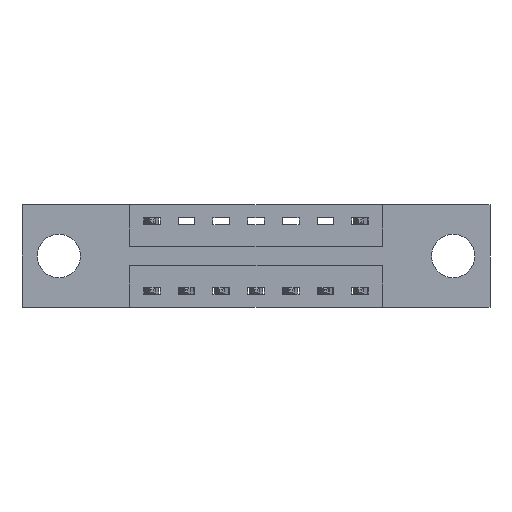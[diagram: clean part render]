
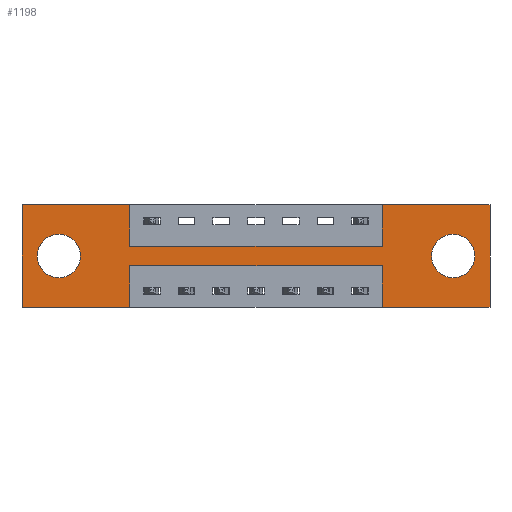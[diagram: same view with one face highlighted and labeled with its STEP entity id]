
A CAD part, front view. The second image highlights one B-rep face of the part: STEP entity #1198.
In plain terms, the highlighted planar face has unit normal (0, -1, 0).
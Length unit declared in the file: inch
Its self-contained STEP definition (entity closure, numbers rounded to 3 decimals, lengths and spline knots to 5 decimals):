
#20 = CARTESIAN_POINT ( 'NONE',  ( 1.5525, 0., -0.185 ) ) ;
#80 = CARTESIAN_POINT ( 'NONE',  ( 0.3875, 0., 0. ) ) ;
#141 = FACE_BOUND ( 'NONE', #5571, .T. ) ;
#266 = EDGE_LOOP ( 'NONE', ( #6934, #7665, #6947, #8512, #7149, #7156, #8659, #7692, #7305, #8444, #7357, #8409 ) ) ;
#296 = DIRECTION ( 'NONE',  ( 0., 1., 0. ) ) ;
#510 = LINE ( 'NONE', #8257, #4146 ) ;
#536 = DIRECTION ( 'NONE',  ( -1., 0., 0. ) ) ;
#577 = VERTEX_POINT ( 'NONE', #8820 ) ;
#596 = LINE ( 'NONE', #5218, #8193 ) ;
#825 = AXIS2_PLACEMENT_3D ( 'NONE', #4644, #296, #5384 ) ;
#826 = DIRECTION ( 'NONE',  ( 0., 0., -1. ) ) ;
#847 = EDGE_CURVE ( 'NONE', #7446, #1345, #1660, .T. ) ;
#893 = DIRECTION ( 'NONE',  ( 0., 0., -1. ) ) ;
#1031 = CARTESIAN_POINT ( 'NONE',  ( 1.2975, 0., -0.22 ) ) ;
#1149 = VERTEX_POINT ( 'NONE', #3296 ) ;
#1194 = EDGE_CURVE ( 'NONE', #7522, #4531, #8883, .T. ) ;
#1198 = ADVANCED_FACE ( 'NONE', ( #141, #7212, #3389 ), #7716, .T. ) ;
#1345 = VERTEX_POINT ( 'NONE', #2401 ) ;
#1363 = DIRECTION ( 'NONE',  ( 0., -1., 0. ) ) ;
#1406 = VECTOR ( 'NONE', #2763, 39.37008 ) ;
#1538 = EDGE_CURVE ( 'NONE', #577, #3326, #7720, .T. ) ;
#1622 = CARTESIAN_POINT ( 'NONE',  ( 0.3875, 0., -0.15 ) ) ;
#1660 = CIRCLE ( 'NONE', #1669, 0.078 ) ;
#1669 = AXIS2_PLACEMENT_3D ( 'NONE', #3978, #8791, #4691 ) ;
#1835 = DIRECTION ( 'NONE',  ( -1., 0., 0. ) ) ;
#2041 = AXIS2_PLACEMENT_3D ( 'NONE', #4094, #8903, #4811 ) ;
#2159 = LINE ( 'NONE', #3451, #5733 ) ;
#2330 = EDGE_CURVE ( 'NONE', #5428, #7073, #5741, .T. ) ;
#2401 = CARTESIAN_POINT ( 'NONE',  ( 0.1325, 0., -0.263 ) ) ;
#2444 = VECTOR ( 'NONE', #1835, 39.37008 ) ;
#2590 = EDGE_CURVE ( 'NONE', #1149, #577, #7704, .T. ) ;
#2673 = AXIS2_PLACEMENT_3D ( 'NONE', #20, #5143, #826 ) ;
#2737 = EDGE_CURVE ( 'NONE', #1345, #7446, #2800, .T. ) ;
#2741 = DIRECTION ( 'NONE',  ( 1., 0., 0. ) ) ;
#2761 = LINE ( 'NONE', #7681, #6616 ) ;
#2763 = DIRECTION ( 'NONE',  ( 0., 0., 1. ) ) ;
#2771 = CARTESIAN_POINT ( 'NONE',  ( 0.3875, 0., -0.37 ) ) ;
#2800 = CIRCLE ( 'NONE', #2041, 0.078 ) ;
#2839 = EDGE_CURVE ( 'NONE', #5321, #1149, #2159, .T. ) ;
#3107 = VERTEX_POINT ( 'NONE', #3973 ) ;
#3231 = LINE ( 'NONE', #6385, #6422 ) ;
#3259 = LINE ( 'NONE', #8984, #1406 ) ;
#3270 = CARTESIAN_POINT ( 'NONE',  ( 1.5525, 0., -0.107 ) ) ;
#3296 = CARTESIAN_POINT ( 'NONE',  ( 1.685, 0., 0. ) ) ;
#3326 = VERTEX_POINT ( 'NONE', #8372 ) ;
#3389 = FACE_OUTER_BOUND ( 'NONE', #266, .T. ) ;
#3451 = CARTESIAN_POINT ( 'NONE',  ( 0., 0., 0. ) ) ;
#3539 = CARTESIAN_POINT ( 'NONE',  ( 0., 0., 0. ) ) ;
#3608 = CIRCLE ( 'NONE', #825, 0.078 ) ;
#3642 = VECTOR ( 'NONE', #8021, 39.37008 ) ;
#3737 = VERTEX_POINT ( 'NONE', #6103 ) ;
#3743 = EDGE_CURVE ( 'NONE', #7073, #5428, #3608, .T. ) ;
#3852 = CARTESIAN_POINT ( 'NONE',  ( 1.5525, 0., -0.263 ) ) ;
#3913 = EDGE_CURVE ( 'NONE', #4167, #8632, #510, .T. ) ;
#3969 = CARTESIAN_POINT ( 'NONE',  ( 1.685, 0., 0. ) ) ;
#3973 = CARTESIAN_POINT ( 'NONE',  ( 1.2975, 0., -0.15 ) ) ;
#3978 = CARTESIAN_POINT ( 'NONE',  ( 0.1325, 0., -0.185 ) ) ;
#4094 = CARTESIAN_POINT ( 'NONE',  ( 0.1325, 0., -0.185 ) ) ;
#4100 = EDGE_CURVE ( 'NONE', #3326, #5929, #3259, .T. ) ;
#4131 = CARTESIAN_POINT ( 'NONE',  ( 0.1325, 0., -0.107 ) ) ;
#4146 = VECTOR ( 'NONE', #4772, 39.37008 ) ;
#4167 = VERTEX_POINT ( 'NONE', #3539 ) ;
#4308 = LINE ( 'NONE', #4608, #2444 ) ;
#4531 = VERTEX_POINT ( 'NONE', #5911 ) ;
#4608 = CARTESIAN_POINT ( 'NONE',  ( 0.3875, 0., -0.22 ) ) ;
#4644 = CARTESIAN_POINT ( 'NONE',  ( 1.5525, 0., -0.185 ) ) ;
#4691 = DIRECTION ( 'NONE',  ( 0., 0., 1. ) ) ;
#4772 = DIRECTION ( 'NONE',  ( 1., 0., 0. ) ) ;
#4811 = DIRECTION ( 'NONE',  ( 0., 0., 1. ) ) ;
#4864 = CARTESIAN_POINT ( 'NONE',  ( 0., 0., -0.37 ) ) ;
#4991 = DIRECTION ( 'NONE',  ( -1., 0., 0. ) ) ;
#5143 = DIRECTION ( 'NONE',  ( 0., 1., 0. ) ) ;
#5218 = CARTESIAN_POINT ( 'NONE',  ( 0.3875, 0., -0.15 ) ) ;
#5251 = EDGE_CURVE ( 'NONE', #6412, #3107, #596, .T. ) ;
#5308 = CARTESIAN_POINT ( 'NONE',  ( 1.2975, 0., 0. ) ) ;
#5321 = VERTEX_POINT ( 'NONE', #5308 ) ;
#5384 = DIRECTION ( 'NONE',  ( 0., 0., -1. ) ) ;
#5428 = VERTEX_POINT ( 'NONE', #3270 ) ;
#5561 = LINE ( 'NONE', #7993, #3642 ) ;
#5571 = EDGE_LOOP ( 'NONE', ( #7004, #7495 ) ) ;
#5606 = EDGE_CURVE ( 'NONE', #4531, #4167, #3231, .T. ) ;
#5733 = VECTOR ( 'NONE', #2741, 39.37008 ) ;
#5741 = CIRCLE ( 'NONE', #2673, 0.078 ) ;
#5911 = CARTESIAN_POINT ( 'NONE',  ( 0., 0., -0.37 ) ) ;
#5929 = VERTEX_POINT ( 'NONE', #1031 ) ;
#6103 = CARTESIAN_POINT ( 'NONE',  ( 0.3875, 0., -0.22 ) ) ;
#6332 = VECTOR ( 'NONE', #4991, 39.37008 ) ;
#6377 = DIRECTION ( 'NONE',  ( 0., 0., -1. ) ) ;
#6385 = CARTESIAN_POINT ( 'NONE',  ( 0., 0., 0. ) ) ;
#6412 = VERTEX_POINT ( 'NONE', #1622 ) ;
#6422 = VECTOR ( 'NONE', #7085, 39.37008 ) ;
#6511 = EDGE_LOOP ( 'NONE', ( #6904, #7629 ) ) ;
#6536 = AXIS2_PLACEMENT_3D ( 'NONE', #8343, #1363, #6377 ) ;
#6616 = VECTOR ( 'NONE', #8926, 39.37008 ) ;
#6904 = ORIENTED_EDGE ( 'NONE', *, *, #847, .T. ) ;
#6934 = ORIENTED_EDGE ( 'NONE', *, *, #8989, .F. ) ;
#6947 = ORIENTED_EDGE ( 'NONE', *, *, #4100, .F. ) ;
#7004 = ORIENTED_EDGE ( 'NONE', *, *, #2330, .T. ) ;
#7073 = VERTEX_POINT ( 'NONE', #3852 ) ;
#7085 = DIRECTION ( 'NONE',  ( 0., 0., 1. ) ) ;
#7149 = ORIENTED_EDGE ( 'NONE', *, *, #2590, .F. ) ;
#7156 = ORIENTED_EDGE ( 'NONE', *, *, #2839, .F. ) ;
#7212 = FACE_BOUND ( 'NONE', #6511, .T. ) ;
#7305 = ORIENTED_EDGE ( 'NONE', *, *, #7963, .F. ) ;
#7357 = ORIENTED_EDGE ( 'NONE', *, *, #5606, .F. ) ;
#7409 = VECTOR ( 'NONE', #536, 39.37008 ) ;
#7446 = VERTEX_POINT ( 'NONE', #4131 ) ;
#7480 = VECTOR ( 'NONE', #8761, 39.37008 ) ;
#7495 = ORIENTED_EDGE ( 'NONE', *, *, #3743, .T. ) ;
#7522 = VERTEX_POINT ( 'NONE', #2771 ) ;
#7554 = VECTOR ( 'NONE', #893, 39.37008 ) ;
#7629 = ORIENTED_EDGE ( 'NONE', *, *, #2737, .T. ) ;
#7665 = ORIENTED_EDGE ( 'NONE', *, *, #8166, .F. ) ;
#7681 = CARTESIAN_POINT ( 'NONE',  ( 1.2975, 0., 0. ) ) ;
#7692 = ORIENTED_EDGE ( 'NONE', *, *, #5251, .F. ) ;
#7704 = LINE ( 'NONE', #3969, #7480 ) ;
#7716 = PLANE ( 'NONE',  #6536 ) ;
#7720 = LINE ( 'NONE', #9057, #6332 ) ;
#7775 = LINE ( 'NONE', #80, #7554 ) ;
#7795 = CARTESIAN_POINT ( 'NONE',  ( 0.3875, 0., 0. ) ) ;
#7963 = EDGE_CURVE ( 'NONE', #8632, #6412, #7775, .T. ) ;
#7993 = CARTESIAN_POINT ( 'NONE',  ( 0.3875, 0., -0.37 ) ) ;
#8021 = DIRECTION ( 'NONE',  ( 0., 0., -1. ) ) ;
#8166 = EDGE_CURVE ( 'NONE', #5929, #3737, #4308, .T. ) ;
#8193 = VECTOR ( 'NONE', #8633, 39.37008 ) ;
#8257 = CARTESIAN_POINT ( 'NONE',  ( 0., 0., 0. ) ) ;
#8343 = CARTESIAN_POINT ( 'NONE',  ( 0., 0., -0.37 ) ) ;
#8372 = CARTESIAN_POINT ( 'NONE',  ( 1.2975, 0., -0.37 ) ) ;
#8409 = ORIENTED_EDGE ( 'NONE', *, *, #1194, .F. ) ;
#8444 = ORIENTED_EDGE ( 'NONE', *, *, #3913, .F. ) ;
#8465 = EDGE_CURVE ( 'NONE', #3107, #5321, #2761, .T. ) ;
#8512 = ORIENTED_EDGE ( 'NONE', *, *, #1538, .F. ) ;
#8632 = VERTEX_POINT ( 'NONE', #7795 ) ;
#8633 = DIRECTION ( 'NONE',  ( 1., 0., 0. ) ) ;
#8659 = ORIENTED_EDGE ( 'NONE', *, *, #8465, .F. ) ;
#8761 = DIRECTION ( 'NONE',  ( 0., 0., -1. ) ) ;
#8791 = DIRECTION ( 'NONE',  ( 0., 1., 0. ) ) ;
#8820 = CARTESIAN_POINT ( 'NONE',  ( 1.685, 0., -0.37 ) ) ;
#8883 = LINE ( 'NONE', #4864, #7409 ) ;
#8903 = DIRECTION ( 'NONE',  ( 0., 1., 0. ) ) ;
#8926 = DIRECTION ( 'NONE',  ( 0., 0., 1. ) ) ;
#8984 = CARTESIAN_POINT ( 'NONE',  ( 1.2975, 0., -0.37 ) ) ;
#8989 = EDGE_CURVE ( 'NONE', #3737, #7522, #5561, .T. ) ;
#9057 = CARTESIAN_POINT ( 'NONE',  ( 0., 0., -0.37 ) ) ;
